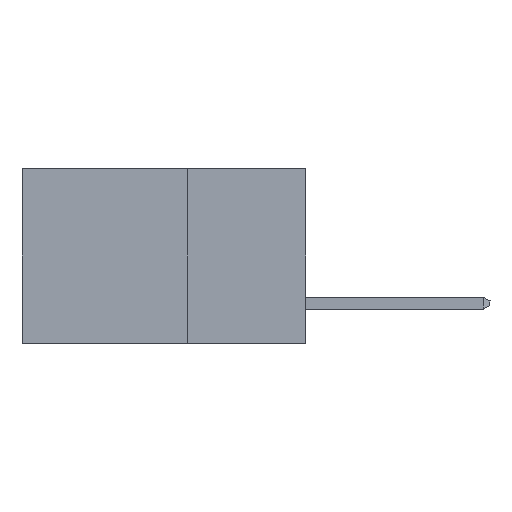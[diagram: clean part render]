
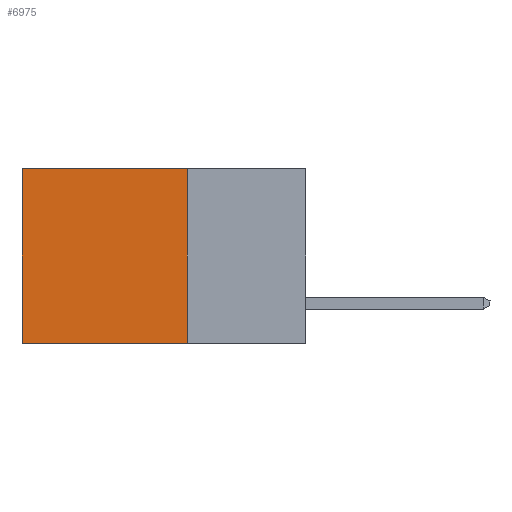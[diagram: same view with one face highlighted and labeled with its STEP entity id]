
A CAD part, left-side view. The second image highlights one B-rep face of the part: STEP entity #6975.
In plain terms, the highlighted planar face has unit normal (-1, 0, 0).
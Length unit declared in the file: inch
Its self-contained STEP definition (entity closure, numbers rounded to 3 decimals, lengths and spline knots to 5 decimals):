
#109 = DIRECTION ( 'NONE',  ( 0., 0., -1. ) ) ;
#1302 = LINE ( 'NONE', #8193, #9192 ) ;
#1440 = FACE_OUTER_BOUND ( 'NONE', #20815, .T. ) ;
#1836 = LINE ( 'NONE', #21679, #10647 ) ;
#3602 = DIRECTION ( 'NONE',  ( 1., 0., 0. ) ) ;
#3735 = EDGE_CURVE ( 'NONE', #18028, #12395, #18279, .T. ) ;
#5114 = ORIENTED_EDGE ( 'NONE', *, *, #15827, .T. ) ;
#5178 = VECTOR ( 'NONE', #109, 39.37008 ) ;
#6975 = ADVANCED_FACE ( 'NONE', ( #1440 ), #13343, .F. ) ;
#7310 = AXIS2_PLACEMENT_3D ( 'NONE', #13015, #3602, #11238 ) ;
#7741 = CARTESIAN_POINT ( 'NONE',  ( 0.298, 0.25, 0. ) ) ;
#8181 = CARTESIAN_POINT ( 'NONE',  ( 0.298, 0.25, 0. ) ) ;
#8193 = CARTESIAN_POINT ( 'NONE',  ( 0.298, 0.6, 0. ) ) ;
#8498 = VERTEX_POINT ( 'NONE', #11960 ) ;
#9192 = VECTOR ( 'NONE', #18002, 39.37008 ) ;
#9843 = ORIENTED_EDGE ( 'NONE', *, *, #18039, .F. ) ;
#10647 = VECTOR ( 'NONE', #15907, 39.37008 ) ;
#11238 = DIRECTION ( 'NONE',  ( 0., 0., -1. ) ) ;
#11960 = CARTESIAN_POINT ( 'NONE',  ( 0.298, 0.25, -0.37 ) ) ;
#12395 = VERTEX_POINT ( 'NONE', #22776 ) ;
#13015 = CARTESIAN_POINT ( 'NONE',  ( 0.298, 0.25, 0. ) ) ;
#13343 = PLANE ( 'NONE',  #7310 ) ;
#13922 = CARTESIAN_POINT ( 'NONE',  ( 0.298, 0.25, 0. ) ) ;
#14194 = CARTESIAN_POINT ( 'NONE',  ( 0.298, 0.6, -0.37 ) ) ;
#14855 = LINE ( 'NONE', #13922, #5178 ) ;
#15048 = VERTEX_POINT ( 'NONE', #14194 ) ;
#15827 = EDGE_CURVE ( 'NONE', #12395, #15048, #1302, .T. ) ;
#15873 = ORIENTED_EDGE ( 'NONE', *, *, #16995, .F. ) ;
#15907 = DIRECTION ( 'NONE',  ( 0., 1., 0. ) ) ;
#16995 = EDGE_CURVE ( 'NONE', #18028, #8498, #14855, .T. ) ;
#17636 = DIRECTION ( 'NONE',  ( 0., 1., 0. ) ) ;
#18002 = DIRECTION ( 'NONE',  ( 0., 0., -1. ) ) ;
#18028 = VERTEX_POINT ( 'NONE', #8181 ) ;
#18039 = EDGE_CURVE ( 'NONE', #8498, #15048, #1836, .T. ) ;
#18279 = LINE ( 'NONE', #7741, #23720 ) ;
#18759 = ORIENTED_EDGE ( 'NONE', *, *, #3735, .T. ) ;
#20815 = EDGE_LOOP ( 'NONE', ( #5114, #9843, #15873, #18759 ) ) ;
#21679 = CARTESIAN_POINT ( 'NONE',  ( 0.298, 0.25, -0.37 ) ) ;
#22776 = CARTESIAN_POINT ( 'NONE',  ( 0.298, 0.6, 0. ) ) ;
#23720 = VECTOR ( 'NONE', #17636, 39.37008 ) ;
